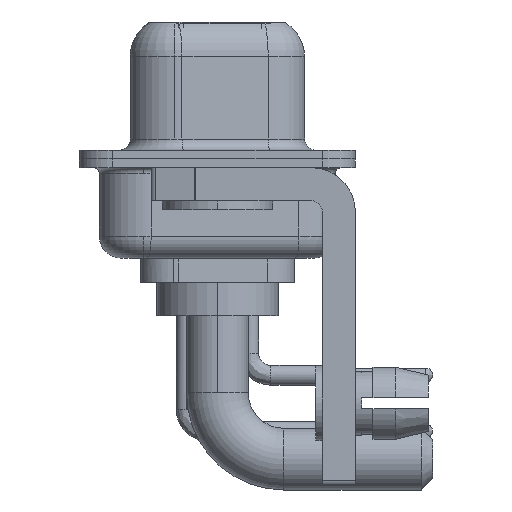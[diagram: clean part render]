
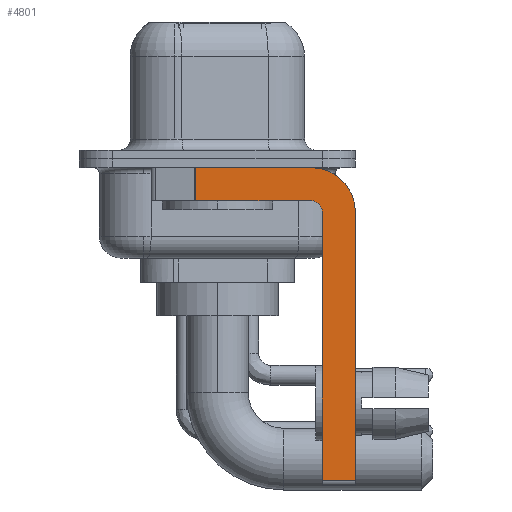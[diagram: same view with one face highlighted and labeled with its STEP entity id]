
A CAD part, left-side view. The second image highlights one B-rep face of the part: STEP entity #4801.
In plain terms, the highlighted planar face has unit normal (-1, 0, 0).
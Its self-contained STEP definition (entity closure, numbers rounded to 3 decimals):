
#316 = VECTOR ( 'NONE', #17746, 1000. ) ;
#1003 = CARTESIAN_POINT ( 'NONE',  ( -2.9, -6.25, -2.4 ) ) ;
#1708 = CARTESIAN_POINT ( 'NONE',  ( -2.9, -4.25, -2.4 ) ) ;
#2688 = AXIS2_PLACEMENT_3D ( 'NONE', #13220, #11500, #9784 ) ;
#3328 = EDGE_CURVE ( 'NONE', #11141, #5415, #3925, .T. ) ;
#3374 = VECTOR ( 'NONE', #21429, 1000. ) ;
#3573 = ORIENTED_EDGE ( 'NONE', *, *, #3328, .F. ) ;
#3650 = DIRECTION ( 'NONE',  ( 0., 0., 1. ) ) ;
#3656 = CARTESIAN_POINT ( 'NONE',  ( -2.9, -4.75, -14.55 ) ) ;
#3923 = VECTOR ( 'NONE', #5126, 1000. ) ;
#3925 = LINE ( 'NONE', #7130, #17910 ) ;
#4066 = DIRECTION ( 'NONE',  ( 0., 0., -1. ) ) ;
#4295 = EDGE_CURVE ( 'NONE', #17596, #5760, #5449, .T. ) ;
#4456 = VERTEX_POINT ( 'NONE', #1003 ) ;
#4801 = ADVANCED_FACE ( 'NONE', ( #22109 ), #16737, .F. ) ;
#5126 = DIRECTION ( 'NONE',  ( 0., -1., 0. ) ) ;
#5170 = EDGE_CURVE ( 'NONE', #18933, #17596, #17628, .T. ) ;
#5250 = EDGE_LOOP ( 'NONE', ( #3573, #5319, #15485, #9609, #22418, #18253, #13723, #11342 ) ) ;
#5319 = ORIENTED_EDGE ( 'NONE', *, *, #15164, .T. ) ;
#5415 = VERTEX_POINT ( 'NONE', #15442 ) ;
#5449 = CIRCLE ( 'NONE', #21896, 0.5 ) ;
#5542 = CARTESIAN_POINT ( 'NONE',  ( -2.9, -6.25, -2.4 ) ) ;
#5760 = VERTEX_POINT ( 'NONE', #14488 ) ;
#5830 = AXIS2_PLACEMENT_3D ( 'NONE', #7809, #21642, #7928 ) ;
#6099 = CARTESIAN_POINT ( 'NONE',  ( -2.9, 0.978, -1.9 ) ) ;
#6510 = VERTEX_POINT ( 'NONE', #8070 ) ;
#7130 = CARTESIAN_POINT ( 'NONE',  ( -2.9, 3., -0.4 ) ) ;
#7577 = VECTOR ( 'NONE', #14341, 1000. ) ;
#7809 = CARTESIAN_POINT ( 'NONE',  ( -2.9, -4.25, -2.4 ) ) ;
#7928 = DIRECTION ( 'NONE',  ( 0., 0., -1. ) ) ;
#8070 = CARTESIAN_POINT ( 'NONE',  ( -2.9, -6.25, -14.55 ) ) ;
#8637 = VERTEX_POINT ( 'NONE', #6099 ) ;
#8679 = DIRECTION ( 'NONE',  ( -1., 0., 0. ) ) ;
#9026 = VECTOR ( 'NONE', #4066, 1000. ) ;
#9609 = ORIENTED_EDGE ( 'NONE', *, *, #4295, .F. ) ;
#9784 = DIRECTION ( 'NONE',  ( 0., 0., -1. ) ) ;
#10793 = CARTESIAN_POINT ( 'NONE',  ( -2.9, -4.25, -1.9 ) ) ;
#11052 = CARTESIAN_POINT ( 'NONE',  ( -2.9, -4.75, -2.4 ) ) ;
#11126 = EDGE_CURVE ( 'NONE', #5415, #4456, #13625, .T. ) ;
#11141 = VERTEX_POINT ( 'NONE', #15638 ) ;
#11342 = ORIENTED_EDGE ( 'NONE', *, *, #11126, .F. ) ;
#11500 = DIRECTION ( 'NONE',  ( 1., 0., 0. ) ) ;
#12181 = CARTESIAN_POINT ( 'NONE',  ( -2.9, -4.25, -14.55 ) ) ;
#13220 = CARTESIAN_POINT ( 'NONE',  ( -2.9, -4.25, -2.4 ) ) ;
#13625 = CIRCLE ( 'NONE', #2688, 2. ) ;
#13723 = ORIENTED_EDGE ( 'NONE', *, *, #16790, .F. ) ;
#14341 = DIRECTION ( 'NONE',  ( 0., 1., 0. ) ) ;
#14488 = CARTESIAN_POINT ( 'NONE',  ( -2.9, -4.25, -1.9 ) ) ;
#14967 = EDGE_CURVE ( 'NONE', #18933, #6510, #20798, .T. ) ;
#15062 = EDGE_CURVE ( 'NONE', #5760, #8637, #18141, .T. ) ;
#15164 = EDGE_CURVE ( 'NONE', #11141, #8637, #19863, .T. ) ;
#15442 = CARTESIAN_POINT ( 'NONE',  ( -2.9, -4.25, -0.4 ) ) ;
#15485 = ORIENTED_EDGE ( 'NONE', *, *, #15062, .F. ) ;
#15638 = CARTESIAN_POINT ( 'NONE',  ( -2.9, 0.978, -0.4 ) ) ;
#16737 = PLANE ( 'NONE',  #5830 ) ;
#16790 = EDGE_CURVE ( 'NONE', #4456, #6510, #18005, .T. ) ;
#17596 = VERTEX_POINT ( 'NONE', #11052 ) ;
#17628 = LINE ( 'NONE', #19573, #316 ) ;
#17746 = DIRECTION ( 'NONE',  ( 0., 0., 1. ) ) ;
#17910 = VECTOR ( 'NONE', #20976, 1000. ) ;
#18005 = LINE ( 'NONE', #5542, #3374 ) ;
#18141 = LINE ( 'NONE', #10793, #7577 ) ;
#18253 = ORIENTED_EDGE ( 'NONE', *, *, #14967, .T. ) ;
#18933 = VERTEX_POINT ( 'NONE', #3656 ) ;
#19573 = CARTESIAN_POINT ( 'NONE',  ( -2.9, -4.75, -14.8 ) ) ;
#19863 = LINE ( 'NONE', #21226, #9026 ) ;
#20798 = LINE ( 'NONE', #12181, #3923 ) ;
#20976 = DIRECTION ( 'NONE',  ( 0., -1., 0. ) ) ;
#21226 = CARTESIAN_POINT ( 'NONE',  ( -2.9, 0.978, -1.9 ) ) ;
#21429 = DIRECTION ( 'NONE',  ( 0., 0., -1. ) ) ;
#21642 = DIRECTION ( 'NONE',  ( 1., 0., 0. ) ) ;
#21896 = AXIS2_PLACEMENT_3D ( 'NONE', #1708, #8679, #3650 ) ;
#22109 = FACE_OUTER_BOUND ( 'NONE', #5250, .T. ) ;
#22418 = ORIENTED_EDGE ( 'NONE', *, *, #5170, .F. ) ;
